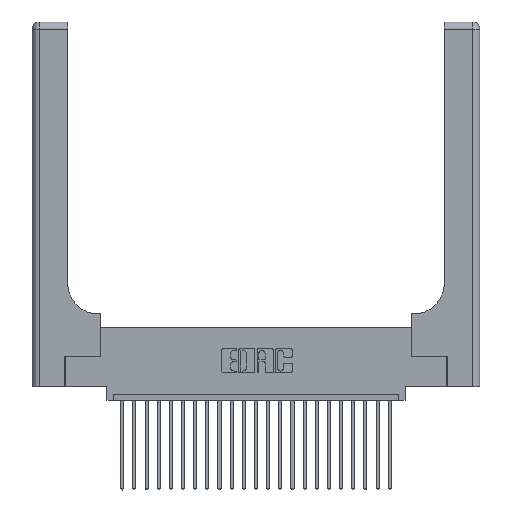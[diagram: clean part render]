
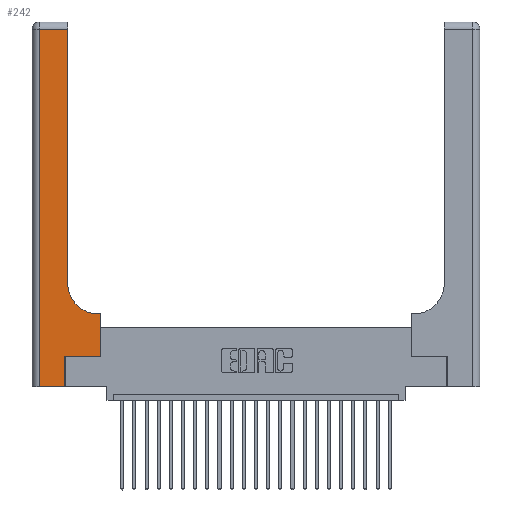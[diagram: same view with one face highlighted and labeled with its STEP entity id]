
A CAD part, top view. The second image highlights one B-rep face of the part: STEP entity #242.
In plain terms, the highlighted planar face has unit normal (0, 0, 1).
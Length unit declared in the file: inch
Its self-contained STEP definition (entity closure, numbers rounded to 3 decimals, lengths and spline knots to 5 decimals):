
#110 = EDGE_LOOP ( 'NONE', ( #23627, #16423, #22665, #20124, #16133, #5864, #21911, #13586, #15817 ) ) ;
#242 = ADVANCED_FACE ( 'NONE', ( #12282 ), #12670, .F. ) ;
#280 = VECTOR ( 'NONE', #11417, 39.37008 ) ;
#375 = CARTESIAN_POINT ( 'NONE',  ( 0.2915, 3., 0.37 ) ) ;
#1041 = CARTESIAN_POINT ( 'NONE',  ( 0., 3., 0.37 ) ) ;
#1260 = CARTESIAN_POINT ( 'NONE',  ( 0.5415, 0.85, 0.37 ) ) ;
#1579 = LINE ( 'NONE', #23114, #10711 ) ;
#1652 = EDGE_CURVE ( 'NONE', #17094, #2222, #24307, .T. ) ;
#2027 = LINE ( 'NONE', #22604, #19682 ) ;
#2222 = VERTEX_POINT ( 'NONE', #7715 ) ;
#2266 = VERTEX_POINT ( 'NONE', #12243 ) ;
#2388 = VERTEX_POINT ( 'NONE', #6538 ) ;
#3034 = DIRECTION ( 'NONE',  ( 0., 1., 0. ) ) ;
#3931 = EDGE_CURVE ( 'NONE', #6039, #2266, #20546, .T. ) ;
#4884 = LINE ( 'NONE', #375, #15835 ) ;
#5228 = DIRECTION ( 'NONE',  ( 0., 0., -1. ) ) ;
#5427 = DIRECTION ( 'NONE',  ( 0., -1., 0. ) ) ;
#5588 = CARTESIAN_POINT ( 'NONE',  ( 0.269, 0.25, 0.37 ) ) ;
#5763 = VECTOR ( 'NONE', #3034, 39.37008 ) ;
#5767 = DIRECTION ( 'NONE',  ( -1., 0., 0. ) ) ;
#5850 = CIRCLE ( 'NONE', #16328, 0.25 ) ;
#5864 = ORIENTED_EDGE ( 'NONE', *, *, #11350, .T. ) ;
#5930 = VERTEX_POINT ( 'NONE', #12669 ) ;
#6039 = VERTEX_POINT ( 'NONE', #9869 ) ;
#6538 = CARTESIAN_POINT ( 'NONE',  ( 0.269, 0., 0.37 ) ) ;
#6931 = DIRECTION ( 'NONE',  ( 0., 0., -1. ) ) ;
#7715 = CARTESIAN_POINT ( 'NONE',  ( 0.5585, 0.6, 0.37 ) ) ;
#8123 = CARTESIAN_POINT ( 'NONE',  ( 0.269, 0., 0.37 ) ) ;
#8311 = EDGE_CURVE ( 'NONE', #23193, #6039, #2027, .T. ) ;
#9349 = CARTESIAN_POINT ( 'NONE',  ( 0.06, 3., 0.37 ) ) ;
#9869 = CARTESIAN_POINT ( 'NONE',  ( 0.06, 2.94, 0.37 ) ) ;
#10230 = VERTEX_POINT ( 'NONE', #5588 ) ;
#10711 = VECTOR ( 'NONE', #5767, 39.37008 ) ;
#10962 = DIRECTION ( 'NONE',  ( 1., 0., 0. ) ) ;
#11350 = EDGE_CURVE ( 'NONE', #10230, #17094, #21333, .T. ) ;
#11417 = DIRECTION ( 'NONE',  ( 1., 0., 0. ) ) ;
#12243 = CARTESIAN_POINT ( 'NONE',  ( 0.06, 0., 0.37 ) ) ;
#12282 = FACE_OUTER_BOUND ( 'NONE', #110, .T. ) ;
#12670 = PLANE ( 'NONE',  #18981 ) ;
#12669 = CARTESIAN_POINT ( 'NONE',  ( 0.5415, 0.6, 0.37 ) ) ;
#13493 = VERTEX_POINT ( 'NONE', #17877 ) ;
#13586 = ORIENTED_EDGE ( 'NONE', *, *, #23895, .T. ) ;
#13769 = DIRECTION ( 'NONE',  ( 0., 1., 0. ) ) ;
#14703 = DIRECTION ( 'NONE',  ( -1., 0., 0. ) ) ;
#14728 = DIRECTION ( 'NONE',  ( -1., 0., 0. ) ) ;
#15377 = LINE ( 'NONE', #8123, #19972 ) ;
#15817 = ORIENTED_EDGE ( 'NONE', *, *, #16856, .T. ) ;
#15835 = VECTOR ( 'NONE', #23670, 39.37008 ) ;
#16133 = ORIENTED_EDGE ( 'NONE', *, *, #20791, .T. ) ;
#16328 = AXIS2_PLACEMENT_3D ( 'NONE', #1260, #5228, #10962 ) ;
#16392 = DIRECTION ( 'NONE',  ( 1., 0., 0. ) ) ;
#16423 = ORIENTED_EDGE ( 'NONE', *, *, #8311, .T. ) ;
#16856 = EDGE_CURVE ( 'NONE', #5930, #13493, #5850, .T. ) ;
#16979 = CARTESIAN_POINT ( 'NONE',  ( 0., 0., 0.37 ) ) ;
#17094 = VERTEX_POINT ( 'NONE', #20756 ) ;
#17877 = CARTESIAN_POINT ( 'NONE',  ( 0.2915, 0.85, 0.37 ) ) ;
#18050 = EDGE_CURVE ( 'NONE', #13493, #23193, #4884, .T. ) ;
#18243 = CARTESIAN_POINT ( 'NONE',  ( 0.269, 0.25, 0.37 ) ) ;
#18261 = LINE ( 'NONE', #16979, #280 ) ;
#18844 = CARTESIAN_POINT ( 'NONE',  ( 0.2915, 2.94, 0.37 ) ) ;
#18981 = AXIS2_PLACEMENT_3D ( 'NONE', #1041, #6931, #14728 ) ;
#19225 = VECTOR ( 'NONE', #16392, 39.37008 ) ;
#19641 = VECTOR ( 'NONE', #5427, 39.37008 ) ;
#19682 = VECTOR ( 'NONE', #14703, 39.37008 ) ;
#19972 = VECTOR ( 'NONE', #13769, 39.37008 ) ;
#20124 = ORIENTED_EDGE ( 'NONE', *, *, #25115, .T. ) ;
#20546 = LINE ( 'NONE', #9349, #19641 ) ;
#20756 = CARTESIAN_POINT ( 'NONE',  ( 0.5585, 0.25, 0.37 ) ) ;
#20791 = EDGE_CURVE ( 'NONE', #2388, #10230, #15377, .T. ) ;
#21333 = LINE ( 'NONE', #18243, #19225 ) ;
#21911 = ORIENTED_EDGE ( 'NONE', *, *, #1652, .T. ) ;
#22565 = CARTESIAN_POINT ( 'NONE',  ( 0.5585, 0.25, 0.37 ) ) ;
#22604 = CARTESIAN_POINT ( 'NONE',  ( 0., 2.94, 0.37 ) ) ;
#22665 = ORIENTED_EDGE ( 'NONE', *, *, #3931, .T. ) ;
#23114 = CARTESIAN_POINT ( 'NONE',  ( 0.2915, 0.6, 0.37 ) ) ;
#23193 = VERTEX_POINT ( 'NONE', #18844 ) ;
#23627 = ORIENTED_EDGE ( 'NONE', *, *, #18050, .T. ) ;
#23670 = DIRECTION ( 'NONE',  ( 0., 1., 0. ) ) ;
#23895 = EDGE_CURVE ( 'NONE', #2222, #5930, #1579, .T. ) ;
#24307 = LINE ( 'NONE', #22565, #5763 ) ;
#25115 = EDGE_CURVE ( 'NONE', #2266, #2388, #18261, .T. ) ;
